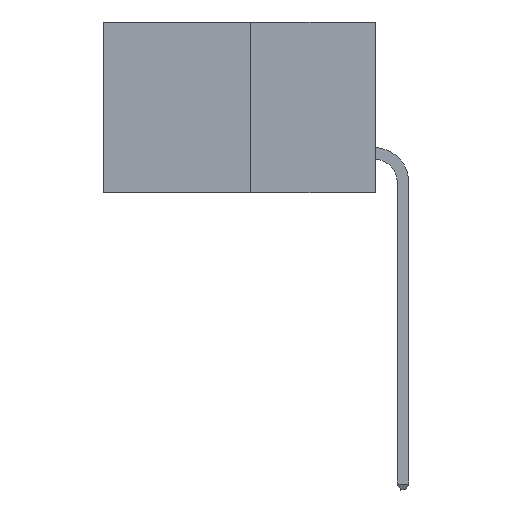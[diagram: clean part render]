
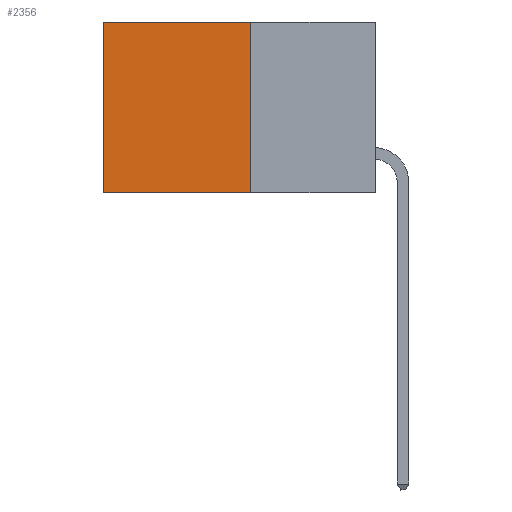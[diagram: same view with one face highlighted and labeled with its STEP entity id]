
A CAD part, left-side view. The second image highlights one B-rep face of the part: STEP entity #2356.
In plain terms, the highlighted planar face has unit normal (-1, 0, 0).
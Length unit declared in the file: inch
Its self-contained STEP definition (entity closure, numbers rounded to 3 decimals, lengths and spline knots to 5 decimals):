
#68 = VECTOR ( 'NONE', #13112, 39.37008 ) ;
#810 = EDGE_CURVE ( 'NONE', #6863, #5966, #3570, .T. ) ;
#1654 = CARTESIAN_POINT ( 'NONE',  ( 0.277, 0.27, -0.37 ) ) ;
#2156 = EDGE_LOOP ( 'NONE', ( #14543, #3241, #12291, #13536 ) ) ;
#2356 = ADVANCED_FACE ( 'NONE', ( #6897 ), #7821, .F. ) ;
#2678 = CARTESIAN_POINT ( 'NONE',  ( 0.277, 0.27, -0.37 ) ) ;
#2985 = EDGE_CURVE ( 'NONE', #6863, #13391, #6861, .T. ) ;
#3241 = ORIENTED_EDGE ( 'NONE', *, *, #12592, .F. ) ;
#3429 = DIRECTION ( 'NONE',  ( 0., 0., -1. ) ) ;
#3432 = EDGE_CURVE ( 'NONE', #13391, #10784, #14374, .T. ) ;
#3570 = LINE ( 'NONE', #2678, #12760 ) ;
#4521 = LINE ( 'NONE', #15252, #8131 ) ;
#4861 = VECTOR ( 'NONE', #3429, 39.37008 ) ;
#5966 = VERTEX_POINT ( 'NONE', #1654 ) ;
#6042 = CARTESIAN_POINT ( 'NONE',  ( 0.277, 0.27, 0. ) ) ;
#6861 = LINE ( 'NONE', #6042, #68 ) ;
#6863 = VERTEX_POINT ( 'NONE', #6896 ) ;
#6896 = CARTESIAN_POINT ( 'NONE',  ( 0.277, 0.27, 0. ) ) ;
#6897 = FACE_OUTER_BOUND ( 'NONE', #2156, .T. ) ;
#7454 = CARTESIAN_POINT ( 'NONE',  ( 0.277, 0.59, 0. ) ) ;
#7534 = DIRECTION ( 'NONE',  ( 0., 0., -1. ) ) ;
#7821 = PLANE ( 'NONE',  #8069 ) ;
#8069 = AXIS2_PLACEMENT_3D ( 'NONE', #9575, #10335, #10391 ) ;
#8131 = VECTOR ( 'NONE', #8174, 39.37008 ) ;
#8174 = DIRECTION ( 'NONE',  ( 0., 1., 0. ) ) ;
#9575 = CARTESIAN_POINT ( 'NONE',  ( 0.277, 0.27, -0.37 ) ) ;
#10335 = DIRECTION ( 'NONE',  ( 1., 0., 0. ) ) ;
#10391 = DIRECTION ( 'NONE',  ( 0., 0., -1. ) ) ;
#10784 = VERTEX_POINT ( 'NONE', #12021 ) ;
#12021 = CARTESIAN_POINT ( 'NONE',  ( 0.277, 0.59, -0.37 ) ) ;
#12291 = ORIENTED_EDGE ( 'NONE', *, *, #810, .F. ) ;
#12592 = EDGE_CURVE ( 'NONE', #5966, #10784, #4521, .T. ) ;
#12760 = VECTOR ( 'NONE', #7534, 39.37008 ) ;
#13112 = DIRECTION ( 'NONE',  ( 0., 1., 0. ) ) ;
#13391 = VERTEX_POINT ( 'NONE', #7454 ) ;
#13536 = ORIENTED_EDGE ( 'NONE', *, *, #2985, .T. ) ;
#14374 = LINE ( 'NONE', #14635, #4861 ) ;
#14543 = ORIENTED_EDGE ( 'NONE', *, *, #3432, .T. ) ;
#14635 = CARTESIAN_POINT ( 'NONE',  ( 0.277, 0.59, -0.37 ) ) ;
#15252 = CARTESIAN_POINT ( 'NONE',  ( 0.277, 0.27, -0.37 ) ) ;
